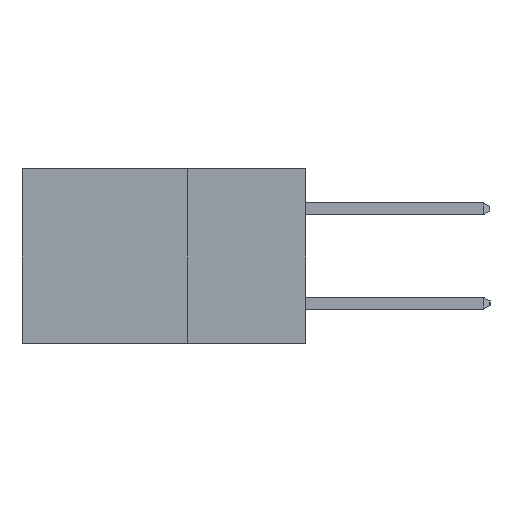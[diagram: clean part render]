
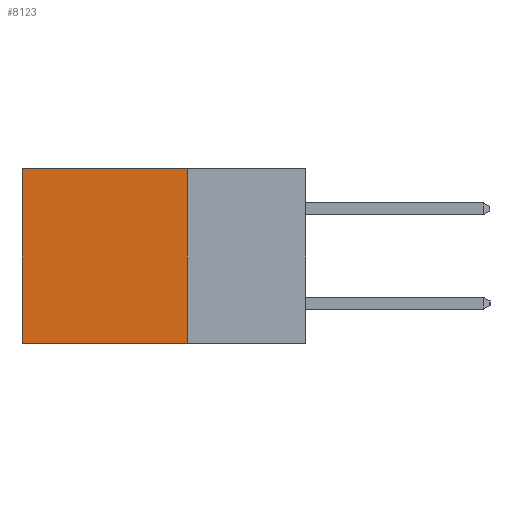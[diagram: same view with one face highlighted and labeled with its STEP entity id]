
A CAD part, left-side view. The second image highlights one B-rep face of the part: STEP entity #8123.
In plain terms, the highlighted planar face has unit normal (-1, 0, 0).
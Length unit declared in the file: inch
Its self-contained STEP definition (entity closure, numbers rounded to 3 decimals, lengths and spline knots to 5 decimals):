
#249 = VECTOR ( 'NONE', #6314, 39.37008 ) ;
#263 = VECTOR ( 'NONE', #3198, 39.37008 ) ;
#575 = ORIENTED_EDGE ( 'NONE', *, *, #7418, .F. ) ;
#2662 = CARTESIAN_POINT ( 'NONE',  ( 0.2615, 0.25, -0.37 ) ) ;
#3131 = VECTOR ( 'NONE', #4900, 39.37008 ) ;
#3151 = EDGE_CURVE ( 'NONE', #10710, #10213, #13782, .T. ) ;
#3198 = DIRECTION ( 'NONE',  ( 0., 1., 0. ) ) ;
#3522 = CARTESIAN_POINT ( 'NONE',  ( 0.2615, 0.6, -0.37 ) ) ;
#3594 = VERTEX_POINT ( 'NONE', #14707 ) ;
#4900 = DIRECTION ( 'NONE',  ( 0., 0., -1. ) ) ;
#5364 = DIRECTION ( 'NONE',  ( 1., 0., 0. ) ) ;
#6314 = DIRECTION ( 'NONE',  ( 0., 0., -1. ) ) ;
#6449 = VECTOR ( 'NONE', #6503, 39.37008 ) ;
#6503 = DIRECTION ( 'NONE',  ( 0., 1., 0. ) ) ;
#6689 = ORIENTED_EDGE ( 'NONE', *, *, #3151, .F. ) ;
#6720 = LINE ( 'NONE', #3522, #3131 ) ;
#7418 = EDGE_CURVE ( 'NONE', #10213, #15757, #7536, .T. ) ;
#7465 = CARTESIAN_POINT ( 'NONE',  ( 0.2615, 0.25, -0.37 ) ) ;
#7536 = LINE ( 'NONE', #2662, #263 ) ;
#8123 = ADVANCED_FACE ( 'NONE', ( #16165 ), #13326, .F. ) ;
#8129 = CARTESIAN_POINT ( 'NONE',  ( 0.2615, 0.6, -0.37 ) ) ;
#9485 = EDGE_LOOP ( 'NONE', ( #12309, #575, #6689, #16740 ) ) ;
#10213 = VERTEX_POINT ( 'NONE', #12206 ) ;
#10710 = VERTEX_POINT ( 'NONE', #11836 ) ;
#11836 = CARTESIAN_POINT ( 'NONE',  ( 0.2615, 0.25, 0. ) ) ;
#12206 = CARTESIAN_POINT ( 'NONE',  ( 0.2615, 0.25, -0.37 ) ) ;
#12309 = ORIENTED_EDGE ( 'NONE', *, *, #17289, .T. ) ;
#13326 = PLANE ( 'NONE',  #14769 ) ;
#13782 = LINE ( 'NONE', #7465, #249 ) ;
#14437 = CARTESIAN_POINT ( 'NONE',  ( 0.2615, 0.25, 0. ) ) ;
#14627 = DIRECTION ( 'NONE',  ( 0., 0., -1. ) ) ;
#14707 = CARTESIAN_POINT ( 'NONE',  ( 0.2615, 0.6, 0. ) ) ;
#14769 = AXIS2_PLACEMENT_3D ( 'NONE', #17101, #5364, #14627 ) ;
#15560 = EDGE_CURVE ( 'NONE', #10710, #3594, #16514, .T. ) ;
#15757 = VERTEX_POINT ( 'NONE', #8129 ) ;
#16165 = FACE_OUTER_BOUND ( 'NONE', #9485, .T. ) ;
#16514 = LINE ( 'NONE', #14437, #6449 ) ;
#16740 = ORIENTED_EDGE ( 'NONE', *, *, #15560, .T. ) ;
#17101 = CARTESIAN_POINT ( 'NONE',  ( 0.2615, 0.25, -0.37 ) ) ;
#17289 = EDGE_CURVE ( 'NONE', #3594, #15757, #6720, .T. ) ;
